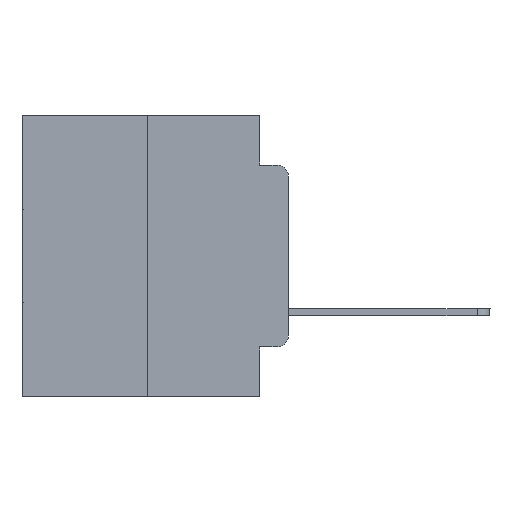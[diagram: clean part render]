
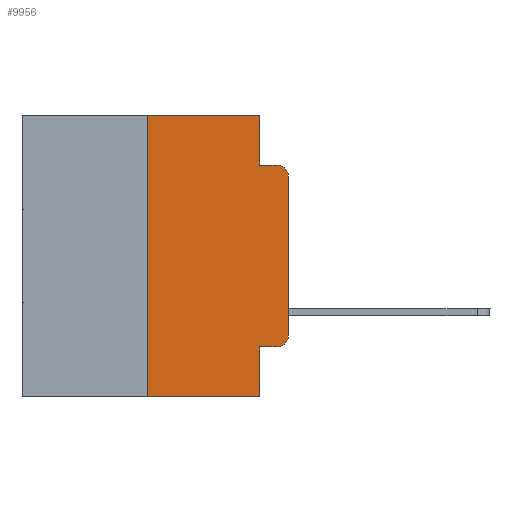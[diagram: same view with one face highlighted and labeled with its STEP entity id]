
A CAD part, left-side view. The second image highlights one B-rep face of the part: STEP entity #9956.
In plain terms, the highlighted planar face has unit normal (-1, 0, 0).
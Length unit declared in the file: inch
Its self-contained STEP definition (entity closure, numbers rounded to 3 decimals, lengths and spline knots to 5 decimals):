
#620 = VECTOR ( 'NONE', #18810, 39.37008 ) ;
#732 = CARTESIAN_POINT ( 'NONE',  ( 0., 0.02, -0.3915 ) ) ;
#1352 = VERTEX_POINT ( 'NONE', #8524 ) ;
#1366 = AXIS2_PLACEMENT_3D ( 'NONE', #732, #11430, #7340 ) ;
#1931 = VERTEX_POINT ( 'NONE', #14195 ) ;
#2039 = CARTESIAN_POINT ( 'NONE',  ( 0., 0.02, -0.4115 ) ) ;
#2146 = CARTESIAN_POINT ( 'NONE',  ( 0., 0.25, -0.5 ) ) ;
#2161 = ORIENTED_EDGE ( 'NONE', *, *, #23765, .T. ) ;
#2162 = VERTEX_POINT ( 'NONE', #10499 ) ;
#2459 = VECTOR ( 'NONE', #20589, 39.37008 ) ;
#2826 = EDGE_CURVE ( 'NONE', #1931, #14321, #3249, .T. ) ;
#3249 = LINE ( 'NONE', #22808, #2459 ) ;
#3481 = FACE_OUTER_BOUND ( 'NONE', #14215, .T. ) ;
#3780 = DIRECTION ( 'NONE',  ( 1., 0., 0. ) ) ;
#4210 = VERTEX_POINT ( 'NONE', #25766 ) ;
#4300 = CARTESIAN_POINT ( 'NONE',  ( 0., 0.25, 0. ) ) ;
#4569 = VERTEX_POINT ( 'NONE', #2039 ) ;
#4692 = VERTEX_POINT ( 'NONE', #21886 ) ;
#4927 = CARTESIAN_POINT ( 'NONE',  ( 0., 0.051, -0.4115 ) ) ;
#5389 = VERTEX_POINT ( 'NONE', #20789 ) ;
#5409 = LINE ( 'NONE', #20847, #22847 ) ;
#5499 = EDGE_CURVE ( 'NONE', #1931, #4569, #7265, .T. ) ;
#6207 = VECTOR ( 'NONE', #27945, 39.37008 ) ;
#6493 = ORIENTED_EDGE ( 'NONE', *, *, #27006, .F. ) ;
#6843 = ORIENTED_EDGE ( 'NONE', *, *, #10863, .F. ) ;
#7078 = CARTESIAN_POINT ( 'NONE',  ( 0., 0.473, -0.5 ) ) ;
#7265 = LINE ( 'NONE', #4927, #12797 ) ;
#7340 = DIRECTION ( 'NONE',  ( 0., 0., -1. ) ) ;
#8482 = LINE ( 'NONE', #27002, #21525 ) ;
#8524 = CARTESIAN_POINT ( 'NONE',  ( 0., 0.051, 0. ) ) ;
#9119 = CARTESIAN_POINT ( 'NONE',  ( 0., 0.473, 0. ) ) ;
#9812 = LINE ( 'NONE', #12443, #620 ) ;
#9860 = CIRCLE ( 'NONE', #26321, 0.02 ) ;
#9956 = ADVANCED_FACE ( 'NONE', ( #3481 ), #19892, .F. ) ;
#10499 = CARTESIAN_POINT ( 'NONE',  ( 0., 0.25, 0. ) ) ;
#10863 = EDGE_CURVE ( 'NONE', #1352, #4210, #8482, .T. ) ;
#11430 = DIRECTION ( 'NONE',  ( -1., 0., 0. ) ) ;
#12443 = CARTESIAN_POINT ( 'NONE',  ( 0., 0.051, -0.0885 ) ) ;
#12625 = VERTEX_POINT ( 'NONE', #2146 ) ;
#12797 = VECTOR ( 'NONE', #13851, 39.37008 ) ;
#12836 = ORIENTED_EDGE ( 'NONE', *, *, #19418, .F. ) ;
#12938 = DIRECTION ( 'NONE',  ( 0., 0., 1. ) ) ;
#13417 = VECTOR ( 'NONE', #12938, 39.37008 ) ;
#13851 = DIRECTION ( 'NONE',  ( 0., -1., 0. ) ) ;
#14014 = CIRCLE ( 'NONE', #1366, 0.02 ) ;
#14036 = ORIENTED_EDGE ( 'NONE', *, *, #18976, .F. ) ;
#14195 = CARTESIAN_POINT ( 'NONE',  ( 0., 0.051, -0.4115 ) ) ;
#14215 = EDGE_LOOP ( 'NONE', ( #27406, #25146, #6493, #6843, #12836, #14036, #18611, #14758, #19952, #2161 ) ) ;
#14321 = VERTEX_POINT ( 'NONE', #18425 ) ;
#14758 = ORIENTED_EDGE ( 'NONE', *, *, #2826, .F. ) ;
#16306 = AXIS2_PLACEMENT_3D ( 'NONE', #9119, #3780, #21697 ) ;
#16556 = DIRECTION ( 'NONE',  ( 0., -1., 0. ) ) ;
#17542 = EDGE_CURVE ( 'NONE', #5389, #21760, #23129, .T. ) ;
#18425 = CARTESIAN_POINT ( 'NONE',  ( 0., 0.051, -0.5 ) ) ;
#18537 = LINE ( 'NONE', #7078, #21495 ) ;
#18611 = ORIENTED_EDGE ( 'NONE', *, *, #20812, .T. ) ;
#18810 = DIRECTION ( 'NONE',  ( 0., -1., 0. ) ) ;
#18976 = EDGE_CURVE ( 'NONE', #12625, #2162, #22090, .T. ) ;
#19418 = EDGE_CURVE ( 'NONE', #2162, #1352, #5409, .T. ) ;
#19583 = CARTESIAN_POINT ( 'NONE',  ( 0., 0.02, -0.1085 ) ) ;
#19823 = DIRECTION ( 'NONE',  ( 0., 0., -1. ) ) ;
#19892 = PLANE ( 'NONE',  #16306 ) ;
#19952 = ORIENTED_EDGE ( 'NONE', *, *, #5499, .T. ) ;
#20589 = DIRECTION ( 'NONE',  ( 0., 0., -1. ) ) ;
#20789 = CARTESIAN_POINT ( 'NONE',  ( 0., 0., -0.3915 ) ) ;
#20812 = EDGE_CURVE ( 'NONE', #12625, #14321, #18537, .T. ) ;
#20847 = CARTESIAN_POINT ( 'NONE',  ( 0., 0.473, 0. ) ) ;
#21495 = VECTOR ( 'NONE', #27206, 39.37008 ) ;
#21525 = VECTOR ( 'NONE', #19823, 39.37008 ) ;
#21697 = DIRECTION ( 'NONE',  ( 0., 0., -1. ) ) ;
#21760 = VERTEX_POINT ( 'NONE', #27817 ) ;
#21886 = CARTESIAN_POINT ( 'NONE',  ( 0., 0.02, -0.0885 ) ) ;
#22090 = LINE ( 'NONE', #4300, #13417 ) ;
#22808 = CARTESIAN_POINT ( 'NONE',  ( 0., 0.051, 0. ) ) ;
#22847 = VECTOR ( 'NONE', #16556, 39.37008 ) ;
#23129 = LINE ( 'NONE', #27512, #6207 ) ;
#23765 = EDGE_CURVE ( 'NONE', #4569, #5389, #14014, .T. ) ;
#24810 = EDGE_CURVE ( 'NONE', #21760, #4692, #9860, .T. ) ;
#25146 = ORIENTED_EDGE ( 'NONE', *, *, #24810, .T. ) ;
#25766 = CARTESIAN_POINT ( 'NONE',  ( 0., 0.051, -0.0885 ) ) ;
#26321 = AXIS2_PLACEMENT_3D ( 'NONE', #19583, #26489, #28545 ) ;
#26489 = DIRECTION ( 'NONE',  ( -1., 0., 0. ) ) ;
#27002 = CARTESIAN_POINT ( 'NONE',  ( 0., 0.051, 0. ) ) ;
#27006 = EDGE_CURVE ( 'NONE', #4210, #4692, #9812, .T. ) ;
#27206 = DIRECTION ( 'NONE',  ( 0., -1., 0. ) ) ;
#27406 = ORIENTED_EDGE ( 'NONE', *, *, #17542, .T. ) ;
#27512 = CARTESIAN_POINT ( 'NONE',  ( 0., 0., 0. ) ) ;
#27817 = CARTESIAN_POINT ( 'NONE',  ( 0., 0., -0.1085 ) ) ;
#27945 = DIRECTION ( 'NONE',  ( 0., 0., 1. ) ) ;
#28545 = DIRECTION ( 'NONE',  ( 0., 0., -1. ) ) ;
